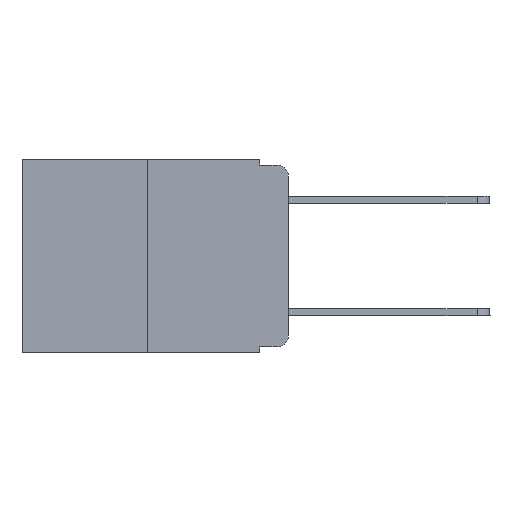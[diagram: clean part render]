
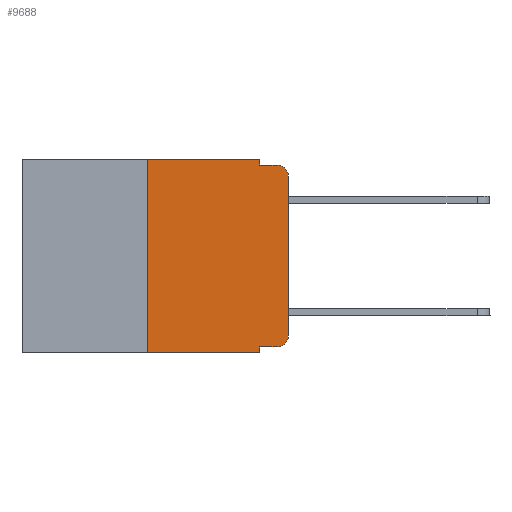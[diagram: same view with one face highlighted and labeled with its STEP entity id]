
A CAD part, left-side view. The second image highlights one B-rep face of the part: STEP entity #9688.
In plain terms, the highlighted planar face has unit normal (-1, 0, 0).
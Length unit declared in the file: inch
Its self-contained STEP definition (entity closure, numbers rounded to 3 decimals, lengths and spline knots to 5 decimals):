
#1116 = VECTOR ( 'NONE', #5064, 39.37008 ) ;
#1274 = VERTEX_POINT ( 'NONE', #13917 ) ;
#1348 = LINE ( 'NONE', #16059, #8116 ) ;
#1436 = DIRECTION ( 'NONE',  ( 0., 0., 1. ) ) ;
#1438 = ORIENTED_EDGE ( 'NONE', *, *, #14107, .T. ) ;
#1521 = AXIS2_PLACEMENT_3D ( 'NONE', #18812, #11216, #12813 ) ;
#1815 = EDGE_CURVE ( 'NONE', #4994, #18744, #1348, .T. ) ;
#2015 = EDGE_LOOP ( 'NONE', ( #17608, #10777, #13149, #18979, #7549, #18197, #5988, #4473, #1438, #4516 ) ) ;
#2410 = DIRECTION ( 'NONE',  ( 0., -1., 0. ) ) ;
#3120 = VERTEX_POINT ( 'NONE', #9473 ) ;
#3509 = CARTESIAN_POINT ( 'NONE',  ( 0., 0., -0.313 ) ) ;
#3931 = VECTOR ( 'NONE', #9252, 39.37008 ) ;
#4473 = ORIENTED_EDGE ( 'NONE', *, *, #12259, .F. ) ;
#4516 = ORIENTED_EDGE ( 'NONE', *, *, #12867, .T. ) ;
#4727 = VERTEX_POINT ( 'NONE', #11723 ) ;
#4819 = VECTOR ( 'NONE', #6552, 39.37008 ) ;
#4864 = LINE ( 'NONE', #12586, #8845 ) ;
#4994 = VERTEX_POINT ( 'NONE', #5280 ) ;
#5064 = DIRECTION ( 'NONE',  ( 0., 0., 1. ) ) ;
#5280 = CARTESIAN_POINT ( 'NONE',  ( 0., 0.25, 0. ) ) ;
#5489 = VERTEX_POINT ( 'NONE', #18474 ) ;
#5743 = VECTOR ( 'NONE', #11495, 39.37008 ) ;
#5988 = ORIENTED_EDGE ( 'NONE', *, *, #13276, .T. ) ;
#6200 = VERTEX_POINT ( 'NONE', #6206 ) ;
#6206 = CARTESIAN_POINT ( 'NONE',  ( 0., 0.02, -0.01 ) ) ;
#6552 = DIRECTION ( 'NONE',  ( 0., -1., 0. ) ) ;
#6657 = CARTESIAN_POINT ( 'NONE',  ( 0., 0.02, -0.313 ) ) ;
#6987 = DIRECTION ( 'NONE',  ( 0., 0., -1. ) ) ;
#7422 = CIRCLE ( 'NONE', #11823, 0.02 ) ;
#7549 = ORIENTED_EDGE ( 'NONE', *, *, #1815, .F. ) ;
#7673 = CARTESIAN_POINT ( 'NONE',  ( 0., 0., 0. ) ) ;
#8116 = VECTOR ( 'NONE', #2410, 39.37008 ) ;
#8272 = CARTESIAN_POINT ( 'NONE',  ( 0., 0.051, -0.01 ) ) ;
#8845 = VECTOR ( 'NONE', #10326, 39.37008 ) ;
#9112 = CARTESIAN_POINT ( 'NONE',  ( 0., 0.02, -0.03 ) ) ;
#9252 = DIRECTION ( 'NONE',  ( 0., -1., 0. ) ) ;
#9473 = CARTESIAN_POINT ( 'NONE',  ( 0., 0.051, -0.343 ) ) ;
#9498 = CARTESIAN_POINT ( 'NONE',  ( 0., 0.051, -0.333 ) ) ;
#9536 = CARTESIAN_POINT ( 'NONE',  ( 0., 0.051, -0.333 ) ) ;
#9645 = PLANE ( 'NONE',  #1521 ) ;
#9650 = CARTESIAN_POINT ( 'NONE',  ( 0., 0., -0.03 ) ) ;
#9688 = ADVANCED_FACE ( 'NONE', ( #14064 ), #9645, .F. ) ;
#10326 = DIRECTION ( 'NONE',  ( 0., 0., -1. ) ) ;
#10397 = LINE ( 'NONE', #8272, #5743 ) ;
#10777 = ORIENTED_EDGE ( 'NONE', *, *, #18692, .T. ) ;
#11008 = CARTESIAN_POINT ( 'NONE',  ( 0., 0.25, 0. ) ) ;
#11031 = DIRECTION ( 'NONE',  ( -1., 0., 0. ) ) ;
#11151 = EDGE_CURVE ( 'NONE', #13283, #13899, #11249, .T. ) ;
#11216 = DIRECTION ( 'NONE',  ( 1., 0., 0. ) ) ;
#11249 = LINE ( 'NONE', #7673, #15211 ) ;
#11495 = DIRECTION ( 'NONE',  ( 0., -1., 0. ) ) ;
#11723 = CARTESIAN_POINT ( 'NONE',  ( 0., 0.02, -0.333 ) ) ;
#11823 = AXIS2_PLACEMENT_3D ( 'NONE', #6657, #11031, #16995 ) ;
#12198 = DIRECTION ( 'NONE',  ( 0., 0., -1. ) ) ;
#12259 = EDGE_CURVE ( 'NONE', #14344, #3120, #13114, .T. ) ;
#12396 = CARTESIAN_POINT ( 'NONE',  ( 0., 0.051, 0. ) ) ;
#12586 = CARTESIAN_POINT ( 'NONE',  ( 0., 0.051, 0. ) ) ;
#12809 = EDGE_CURVE ( 'NONE', #18744, #5489, #4864, .T. ) ;
#12813 = DIRECTION ( 'NONE',  ( 0., 0., -1. ) ) ;
#12867 = EDGE_CURVE ( 'NONE', #4727, #13283, #7422, .T. ) ;
#13114 = LINE ( 'NONE', #14334, #15889 ) ;
#13149 = ORIENTED_EDGE ( 'NONE', *, *, #14685, .F. ) ;
#13276 = EDGE_CURVE ( 'NONE', #1274, #3120, #13973, .T. ) ;
#13283 = VERTEX_POINT ( 'NONE', #3509 ) ;
#13703 = LINE ( 'NONE', #11008, #1116 ) ;
#13899 = VERTEX_POINT ( 'NONE', #9650 ) ;
#13917 = CARTESIAN_POINT ( 'NONE',  ( 0., 0.25, -0.343 ) ) ;
#13973 = LINE ( 'NONE', #15143, #3931 ) ;
#14064 = FACE_OUTER_BOUND ( 'NONE', #2015, .T. ) ;
#14107 = EDGE_CURVE ( 'NONE', #14344, #4727, #14423, .T. ) ;
#14334 = CARTESIAN_POINT ( 'NONE',  ( 0., 0.051, 0. ) ) ;
#14344 = VERTEX_POINT ( 'NONE', #9536 ) ;
#14423 = LINE ( 'NONE', #9498, #4819 ) ;
#14685 = EDGE_CURVE ( 'NONE', #5489, #6200, #10397, .T. ) ;
#14783 = CIRCLE ( 'NONE', #17151, 0.02 ) ;
#15143 = CARTESIAN_POINT ( 'NONE',  ( 0., 0.473, -0.343 ) ) ;
#15211 = VECTOR ( 'NONE', #1436, 39.37008 ) ;
#15889 = VECTOR ( 'NONE', #6987, 39.37008 ) ;
#16059 = CARTESIAN_POINT ( 'NONE',  ( 0., 0.473, 0. ) ) ;
#16413 = EDGE_CURVE ( 'NONE', #1274, #4994, #13703, .T. ) ;
#16995 = DIRECTION ( 'NONE',  ( 0., 0., -1. ) ) ;
#17151 = AXIS2_PLACEMENT_3D ( 'NONE', #9112, #18268, #12198 ) ;
#17608 = ORIENTED_EDGE ( 'NONE', *, *, #11151, .T. ) ;
#18197 = ORIENTED_EDGE ( 'NONE', *, *, #16413, .F. ) ;
#18268 = DIRECTION ( 'NONE',  ( -1., 0., 0. ) ) ;
#18474 = CARTESIAN_POINT ( 'NONE',  ( 0., 0.051, -0.01 ) ) ;
#18692 = EDGE_CURVE ( 'NONE', #13899, #6200, #14783, .T. ) ;
#18744 = VERTEX_POINT ( 'NONE', #12396 ) ;
#18812 = CARTESIAN_POINT ( 'NONE',  ( 0., 0.473, 0. ) ) ;
#18979 = ORIENTED_EDGE ( 'NONE', *, *, #12809, .F. ) ;
